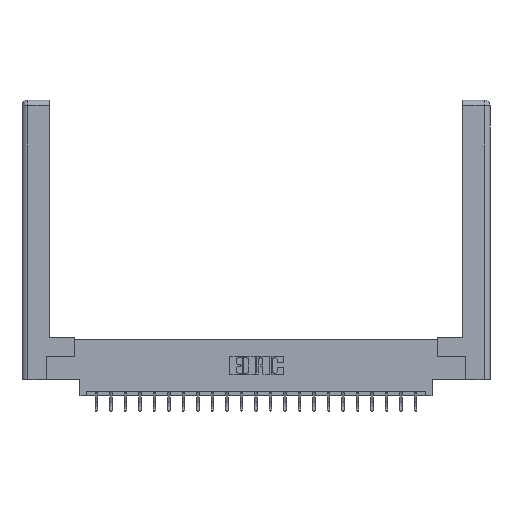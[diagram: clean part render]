
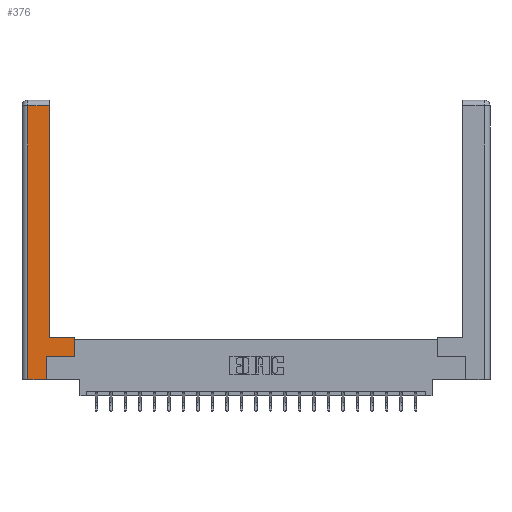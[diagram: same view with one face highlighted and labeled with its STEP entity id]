
A CAD part, top view. The second image highlights one B-rep face of the part: STEP entity #376.
In plain terms, the highlighted planar face has unit normal (0, 0, 1).
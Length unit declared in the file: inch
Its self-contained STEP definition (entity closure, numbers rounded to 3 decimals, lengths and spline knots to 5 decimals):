
#154 = LINE ( 'NONE', #19003, #20421 ) ;
#158 = CARTESIAN_POINT ( 'NONE',  ( 0.565, 0.45, 0. ) ) ;
#376 = ADVANCED_FACE ( 'NONE', ( #23154 ), #3685, .F. ) ;
#553 = VERTEX_POINT ( 'NONE', #9268 ) ;
#754 = VECTOR ( 'NONE', #3143, 39.37008 ) ;
#1055 = ORIENTED_EDGE ( 'NONE', *, *, #15644, .T. ) ;
#1225 = VERTEX_POINT ( 'NONE', #15394 ) ;
#1415 = AXIS2_PLACEMENT_3D ( 'NONE', #5486, #10949, #4380 ) ;
#1421 = LINE ( 'NONE', #7452, #5586 ) ;
#1738 = CARTESIAN_POINT ( 'NONE',  ( 0.0615, 0., 0. ) ) ;
#2392 = DIRECTION ( 'NONE',  ( 0., 1., 0. ) ) ;
#3143 = DIRECTION ( 'NONE',  ( -1., 0., 0. ) ) ;
#3685 = PLANE ( 'NONE',  #1415 ) ;
#4040 = EDGE_CURVE ( 'NONE', #17172, #11230, #13293, .T. ) ;
#4380 = DIRECTION ( 'NONE',  ( -1., 0., 0. ) ) ;
#5056 = CARTESIAN_POINT ( 'NONE',  ( 0.265, 0.245, 0. ) ) ;
#5090 = EDGE_CURVE ( 'NONE', #15781, #553, #1421, .T. ) ;
#5486 = CARTESIAN_POINT ( 'NONE',  ( 0., 0., 0. ) ) ;
#5586 = VECTOR ( 'NONE', #20056, 39.37008 ) ;
#5758 = EDGE_CURVE ( 'NONE', #11230, #15781, #16278, .T. ) ;
#5857 = EDGE_LOOP ( 'NONE', ( #13147, #18256, #1055, #20352, #18863, #14156, #14751, #15902 ) ) ;
#6442 = VECTOR ( 'NONE', #10788, 39.37008 ) ;
#6874 = LINE ( 'NONE', #15694, #19564 ) ;
#7142 = CARTESIAN_POINT ( 'NONE',  ( 0.295, 3., 0. ) ) ;
#7377 = CARTESIAN_POINT ( 'NONE',  ( 0.0615, 0., 0. ) ) ;
#7452 = CARTESIAN_POINT ( 'NONE',  ( 0.565, 0.245, 0. ) ) ;
#7483 = DIRECTION ( 'NONE',  ( 1., 0., 0. ) ) ;
#7849 = EDGE_CURVE ( 'NONE', #553, #17205, #6874, .T. ) ;
#8913 = EDGE_CURVE ( 'NONE', #1225, #17162, #15035, .T. ) ;
#8979 = DIRECTION ( 'NONE',  ( 0., 1., 0. ) ) ;
#9042 = CARTESIAN_POINT ( 'NONE',  ( 0.0615, 2.94, 0. ) ) ;
#9268 = CARTESIAN_POINT ( 'NONE',  ( 0.565, 0.245, 0. ) ) ;
#9985 = DIRECTION ( 'NONE',  ( 0., 1., 0. ) ) ;
#10788 = DIRECTION ( 'NONE',  ( 0., -1., 0. ) ) ;
#10949 = DIRECTION ( 'NONE',  ( 0., 0., -1. ) ) ;
#11180 = VERTEX_POINT ( 'NONE', #9042 ) ;
#11230 = VERTEX_POINT ( 'NONE', #19511 ) ;
#12791 = CARTESIAN_POINT ( 'NONE',  ( 0.265, 0., 0. ) ) ;
#13147 = ORIENTED_EDGE ( 'NONE', *, *, #8913, .T. ) ;
#13293 = LINE ( 'NONE', #12791, #17774 ) ;
#14156 = ORIENTED_EDGE ( 'NONE', *, *, #5090, .T. ) ;
#14324 = EDGE_CURVE ( 'NONE', #17205, #1225, #21569, .T. ) ;
#14751 = ORIENTED_EDGE ( 'NONE', *, *, #7849, .T. ) ;
#15035 = LINE ( 'NONE', #7142, #18695 ) ;
#15394 = CARTESIAN_POINT ( 'NONE',  ( 0.295, 0.45, 0. ) ) ;
#15644 = EDGE_CURVE ( 'NONE', #11180, #17172, #22538, .T. ) ;
#15694 = CARTESIAN_POINT ( 'NONE',  ( 0.565, 0.45, 0. ) ) ;
#15781 = VERTEX_POINT ( 'NONE', #5056 ) ;
#15902 = ORIENTED_EDGE ( 'NONE', *, *, #14324, .T. ) ;
#16278 = LINE ( 'NONE', #16647, #20502 ) ;
#16460 = EDGE_CURVE ( 'NONE', #17162, #11180, #154, .T. ) ;
#16647 = CARTESIAN_POINT ( 'NONE',  ( 0.265, 0.245, 0. ) ) ;
#17162 = VERTEX_POINT ( 'NONE', #17624 ) ;
#17172 = VERTEX_POINT ( 'NONE', #1738 ) ;
#17205 = VERTEX_POINT ( 'NONE', #158 ) ;
#17266 = DIRECTION ( 'NONE',  ( -1., 0., 0. ) ) ;
#17624 = CARTESIAN_POINT ( 'NONE',  ( 0.295, 2.94, 0. ) ) ;
#17774 = VECTOR ( 'NONE', #7483, 39.37008 ) ;
#18256 = ORIENTED_EDGE ( 'NONE', *, *, #16460, .T. ) ;
#18695 = VECTOR ( 'NONE', #8979, 39.37008 ) ;
#18863 = ORIENTED_EDGE ( 'NONE', *, *, #5758, .T. ) ;
#19003 = CARTESIAN_POINT ( 'NONE',  ( 0.0615, 2.94, 0. ) ) ;
#19511 = CARTESIAN_POINT ( 'NONE',  ( 0.265, 0., 0. ) ) ;
#19533 = CARTESIAN_POINT ( 'NONE',  ( 0.295, 0.45, 0. ) ) ;
#19564 = VECTOR ( 'NONE', #9985, 39.37008 ) ;
#20056 = DIRECTION ( 'NONE',  ( 1., 0., 0. ) ) ;
#20352 = ORIENTED_EDGE ( 'NONE', *, *, #4040, .T. ) ;
#20421 = VECTOR ( 'NONE', #17266, 39.37008 ) ;
#20502 = VECTOR ( 'NONE', #2392, 39.37008 ) ;
#21569 = LINE ( 'NONE', #19533, #754 ) ;
#22538 = LINE ( 'NONE', #7377, #6442 ) ;
#23154 = FACE_OUTER_BOUND ( 'NONE', #5857, .T. ) ;
